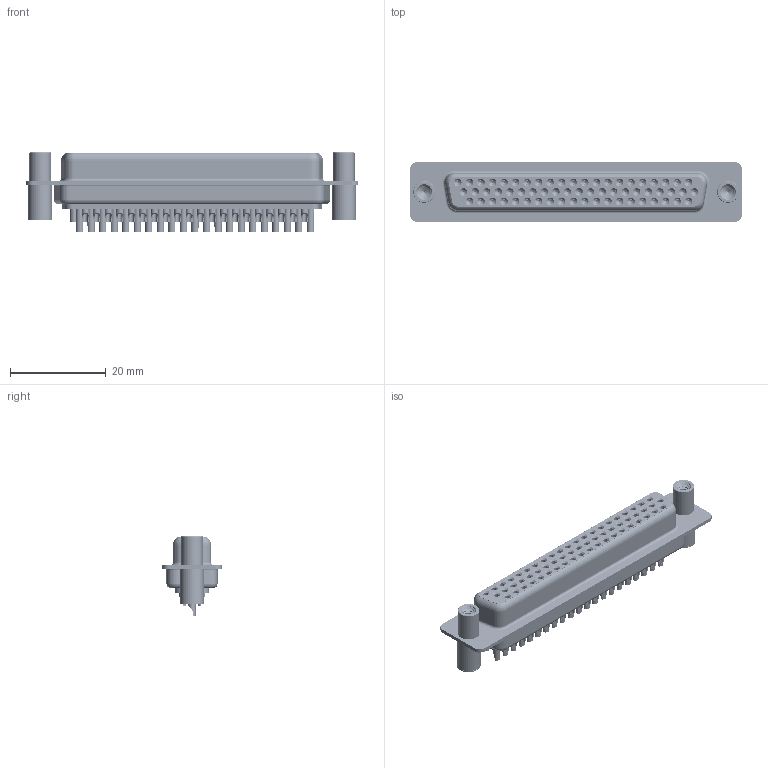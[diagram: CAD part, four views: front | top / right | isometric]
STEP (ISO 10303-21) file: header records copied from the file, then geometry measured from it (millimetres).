
FILE_DESCRIPTION (( 'STEP AP203' ), '1' );
FILE_NAME ('638-M62-232-BN4.STEP', '2022-07-05T21:17:29', ( '' ), ( '' ), 'SwSTEP 2.0', 'SolidWorks 2020', '' );
FILE_SCHEMA (( 'CONFIG_CONTROL_DESIGN' ));
Length unit declared in the file: millimetre
Products named in the file (8): 638-M62-232-BN4; 638M Contact Row 1_32; 638M 4-40 Threaded Standoff and Board Spacer; 638M Shell Front_62 Contacts; 638M Shell Rear_62 Contacts; 638M Contact Row 2_32; 638M Housing_62 Contacts; 638M Contact Row 3_32
Assembly tree (67 placements, depth 2):
  638-M62-232-BN4
    638M Housing_62 Contacts
    638M Shell Front_62 Contacts
    638M Shell Rear_62 Contacts
    638M Contact Row 1_32  x21
    638M Contact Row 2_32  x21
    638M Contact Row 3_32  x20
    638M 4-40 Threaded Standoff and Board Spacer  x2
Bounding box: 69.4 x 12.5 x 16.65 mm (x, y, z)
Volume: 5360.5 mm3; surface area: 17403.3 mm2
Topology: 67 solids, 67 shells, 3775 faces, 9343 edges, 5773 vertices
Faces by surface type: cylinder 1491, plane 1127, cone 588, torus 557, bspline 12
Entity records: 39775 total; most frequent: CARTESIAN_POINT 8408, DIRECTION 6698, ORIENTED_EDGE 5522, AXIS2_PLACEMENT_3D 2836, EDGE_CURVE 2761, VERTEX_POINT 1758, EDGE_LOOP 1561, CIRCLE 1551
